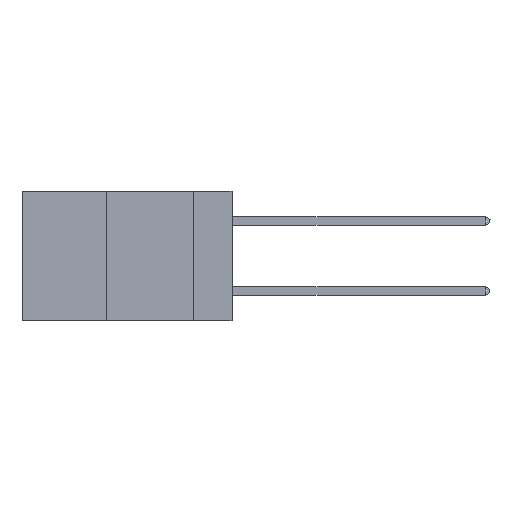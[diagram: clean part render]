
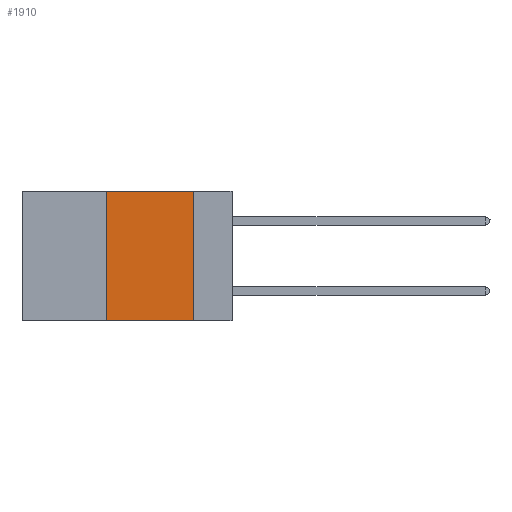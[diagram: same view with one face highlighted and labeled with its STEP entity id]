
A CAD part, left-side view. The second image highlights one B-rep face of the part: STEP entity #1910.
In plain terms, the highlighted planar face has unit normal (-1, 0, 0).
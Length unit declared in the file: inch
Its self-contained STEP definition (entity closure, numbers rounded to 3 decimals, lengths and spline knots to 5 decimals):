
#479 = EDGE_CURVE ( 'NONE', #41917, #38260, #18377, .T. ) ;
#1432 = EDGE_CURVE ( 'NONE', #31240, #2555, #44473, .T. ) ;
#1910 = ADVANCED_FACE ( 'NONE', ( #25992 ), #12138, .F. ) ;
#2555 = VERTEX_POINT ( 'NONE', #22680 ) ;
#3795 = ORIENTED_EDGE ( 'NONE', *, *, #1432, .T. ) ;
#5350 = EDGE_CURVE ( 'NONE', #31240, #41917, #43971, .T. ) ;
#6406 = AXIS2_PLACEMENT_3D ( 'NONE', #24970, #10966, #7179 ) ;
#7179 = DIRECTION ( 'NONE',  ( 0., 0., -1. ) ) ;
#7606 = CARTESIAN_POINT ( 'NONE',  ( 0., 0.6, 0. ) ) ;
#8677 = EDGE_LOOP ( 'NONE', ( #40578, #18246, #17710, #3795 ) ) ;
#8919 = VECTOR ( 'NONE', #34589, 39.37008 ) ;
#9588 = LINE ( 'NONE', #37613, #28289 ) ;
#10966 = DIRECTION ( 'NONE',  ( 1., 0., 0. ) ) ;
#12138 = PLANE ( 'NONE',  #6406 ) ;
#15828 = DIRECTION ( 'NONE',  ( 0., 0., 1. ) ) ;
#16169 = VECTOR ( 'NONE', #15828, 39.37008 ) ;
#16704 = VECTOR ( 'NONE', #20717, 39.37008 ) ;
#17710 = ORIENTED_EDGE ( 'NONE', *, *, #5350, .F. ) ;
#18246 = ORIENTED_EDGE ( 'NONE', *, *, #479, .F. ) ;
#18377 = LINE ( 'NONE', #7606, #8919 ) ;
#20253 = DIRECTION ( 'NONE',  ( 0., 0., -1. ) ) ;
#20717 = DIRECTION ( 'NONE',  ( 0., -1., 0. ) ) ;
#22680 = CARTESIAN_POINT ( 'NONE',  ( 0., 0.11, -0.37 ) ) ;
#23473 = EDGE_CURVE ( 'NONE', #38260, #2555, #9588, .T. ) ;
#23754 = CARTESIAN_POINT ( 'NONE',  ( 0., 0.36, 0. ) ) ;
#24970 = CARTESIAN_POINT ( 'NONE',  ( 0., 0.6, 0. ) ) ;
#25992 = FACE_OUTER_BOUND ( 'NONE', #8677, .T. ) ;
#27798 = CARTESIAN_POINT ( 'NONE',  ( 0., 0.11, 0. ) ) ;
#28289 = VECTOR ( 'NONE', #20253, 39.37008 ) ;
#31240 = VERTEX_POINT ( 'NONE', #33184 ) ;
#33184 = CARTESIAN_POINT ( 'NONE',  ( 0., 0.36, -0.37 ) ) ;
#34589 = DIRECTION ( 'NONE',  ( 0., -1., 0. ) ) ;
#36510 = CARTESIAN_POINT ( 'NONE',  ( 0., 0.6, -0.37 ) ) ;
#36760 = CARTESIAN_POINT ( 'NONE',  ( 0., 0.36, 0. ) ) ;
#37613 = CARTESIAN_POINT ( 'NONE',  ( 0., 0.11, 0. ) ) ;
#38260 = VERTEX_POINT ( 'NONE', #27798 ) ;
#40578 = ORIENTED_EDGE ( 'NONE', *, *, #23473, .F. ) ;
#41917 = VERTEX_POINT ( 'NONE', #23754 ) ;
#43971 = LINE ( 'NONE', #36760, #16169 ) ;
#44473 = LINE ( 'NONE', #36510, #16704 ) ;
